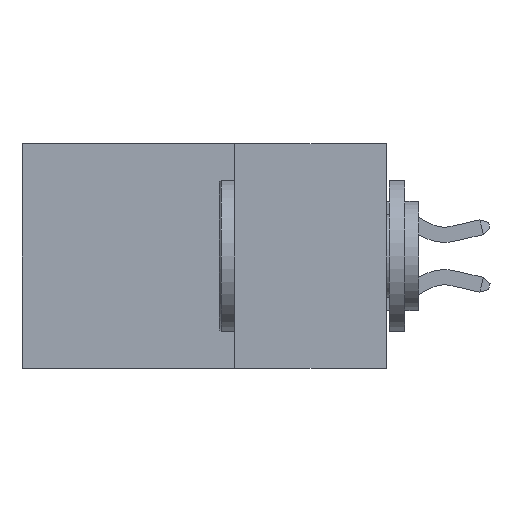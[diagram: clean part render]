
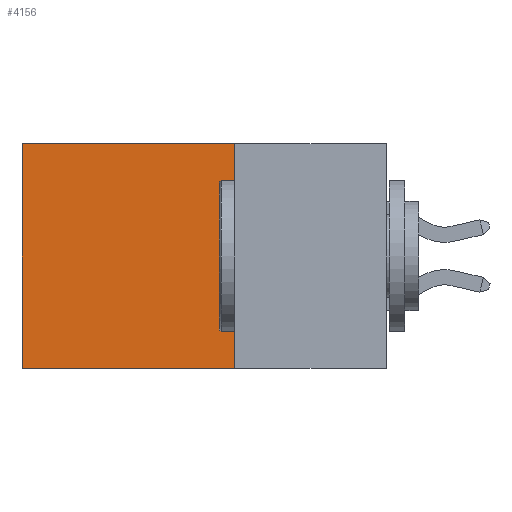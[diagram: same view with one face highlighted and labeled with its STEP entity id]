
A CAD part, left-side view. The second image highlights one B-rep face of the part: STEP entity #4156.
In plain terms, the highlighted planar face has unit normal (-1, 0, 0).
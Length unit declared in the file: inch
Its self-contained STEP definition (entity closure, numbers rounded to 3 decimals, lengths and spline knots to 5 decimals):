
#165 = ORIENTED_EDGE ( 'NONE', *, *, #17611, .F. ) ;
#412 = CARTESIAN_POINT ( 'NONE',  ( 0.2615, 0.6, -0.37 ) ) ;
#3071 = VERTEX_POINT ( 'NONE', #13673 ) ;
#3352 = ORIENTED_EDGE ( 'NONE', *, *, #3662, .T. ) ;
#3662 = EDGE_CURVE ( 'NONE', #3071, #4249, #5604, .T. ) ;
#4156 = ADVANCED_FACE ( 'NONE', ( #10791 ), #12995, .F. ) ;
#4249 = VERTEX_POINT ( 'NONE', #8702 ) ;
#5197 = CARTESIAN_POINT ( 'NONE',  ( 0.2615, 0.25, -0.37 ) ) ;
#5213 = CARTESIAN_POINT ( 'NONE',  ( 0.2615, 0.25, -0.37 ) ) ;
#5604 = LINE ( 'NONE', #6660, #12775 ) ;
#5873 = DIRECTION ( 'NONE',  ( 0., 1., 0. ) ) ;
#6660 = CARTESIAN_POINT ( 'NONE',  ( 0.2615, 0.25, 0. ) ) ;
#7831 = VECTOR ( 'NONE', #12353, 39.37008 ) ;
#8702 = CARTESIAN_POINT ( 'NONE',  ( 0.2615, 0.6, 0. ) ) ;
#9047 = EDGE_CURVE ( 'NONE', #9356, #16809, #16484, .T. ) ;
#9196 = ORIENTED_EDGE ( 'NONE', *, *, #13710, .T. ) ;
#9356 = VERTEX_POINT ( 'NONE', #11622 ) ;
#9587 = DIRECTION ( 'NONE',  ( 0., 0., -1. ) ) ;
#10147 = ORIENTED_EDGE ( 'NONE', *, *, #9047, .F. ) ;
#10791 = FACE_OUTER_BOUND ( 'NONE', #13316, .T. ) ;
#11485 = VECTOR ( 'NONE', #9587, 39.37008 ) ;
#11622 = CARTESIAN_POINT ( 'NONE',  ( 0.2615, 0.25, -0.37 ) ) ;
#11854 = VECTOR ( 'NONE', #15221, 39.37008 ) ;
#12353 = DIRECTION ( 'NONE',  ( 0., 0., -1. ) ) ;
#12775 = VECTOR ( 'NONE', #5873, 39.37008 ) ;
#12907 = DIRECTION ( 'NONE',  ( 0., 0., -1. ) ) ;
#12975 = DIRECTION ( 'NONE',  ( 1., 0., 0. ) ) ;
#12995 = PLANE ( 'NONE',  #15226 ) ;
#13201 = CARTESIAN_POINT ( 'NONE',  ( 0.2615, 0.25, -0.37 ) ) ;
#13316 = EDGE_LOOP ( 'NONE', ( #9196, #10147, #165, #3352 ) ) ;
#13673 = CARTESIAN_POINT ( 'NONE',  ( 0.2615, 0.25, 0. ) ) ;
#13710 = EDGE_CURVE ( 'NONE', #4249, #16809, #14804, .T. ) ;
#14804 = LINE ( 'NONE', #17979, #11485 ) ;
#15221 = DIRECTION ( 'NONE',  ( 0., 1., 0. ) ) ;
#15226 = AXIS2_PLACEMENT_3D ( 'NONE', #13201, #12975, #12907 ) ;
#16484 = LINE ( 'NONE', #5213, #11854 ) ;
#16809 = VERTEX_POINT ( 'NONE', #412 ) ;
#17611 = EDGE_CURVE ( 'NONE', #3071, #9356, #18630, .T. ) ;
#17979 = CARTESIAN_POINT ( 'NONE',  ( 0.2615, 0.6, -0.37 ) ) ;
#18630 = LINE ( 'NONE', #5197, #7831 ) ;
